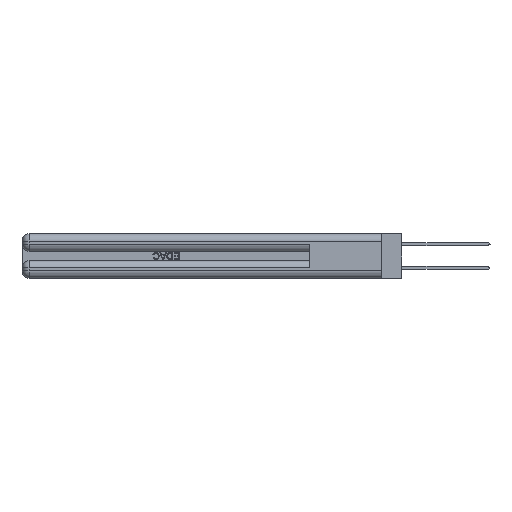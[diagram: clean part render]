
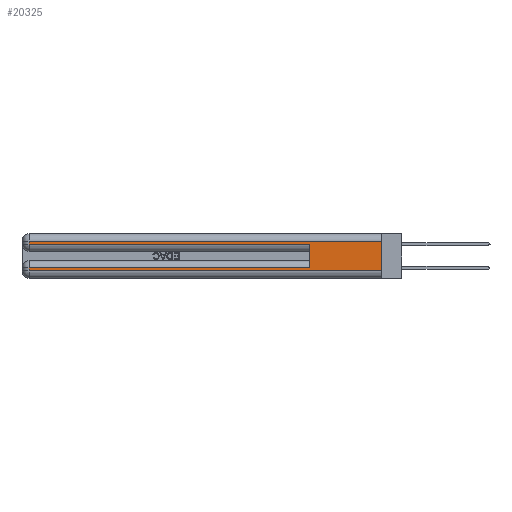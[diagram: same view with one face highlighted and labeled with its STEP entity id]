
A CAD part, left-side view. The second image highlights one B-rep face of the part: STEP entity #20325.
In plain terms, the highlighted planar face has unit normal (-1, 0, 0).
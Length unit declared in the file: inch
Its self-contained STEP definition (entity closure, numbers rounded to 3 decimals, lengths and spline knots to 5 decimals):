
#15 = CARTESIAN_POINT ( 'NONE',  ( 0., 0., 0.06 ) ) ;
#1481 = DIRECTION ( 'NONE',  ( 1., 0., 0. ) ) ;
#1722 = CARTESIAN_POINT ( 'NONE',  ( 0., 2.94, 0.085 ) ) ;
#2175 = LINE ( 'NONE', #39877, #17687 ) ;
#2631 = ORIENTED_EDGE ( 'NONE', *, *, #9699, .T. ) ;
#2966 = DIRECTION ( 'NONE',  ( 0., 1., 0. ) ) ;
#3398 = ORIENTED_EDGE ( 'NONE', *, *, #26807, .T. ) ;
#5607 = VECTOR ( 'NONE', #31214, 39.37008 ) ;
#5855 = ORIENTED_EDGE ( 'NONE', *, *, #34124, .F. ) ;
#5856 = VECTOR ( 'NONE', #18423, 39.37008 ) ;
#6084 = CARTESIAN_POINT ( 'NONE',  ( 0., 0., 0.31 ) ) ;
#6238 = DIRECTION ( 'NONE',  ( 0., 1., 0. ) ) ;
#6672 = ORIENTED_EDGE ( 'NONE', *, *, #23708, .F. ) ;
#8589 = DIRECTION ( 'NONE',  ( 0., -1., 0. ) ) ;
#9699 = EDGE_CURVE ( 'NONE', #20652, #22304, #37117, .T. ) ;
#9713 = EDGE_CURVE ( 'NONE', #44718, #11783, #11287, .T. ) ;
#11287 = LINE ( 'NONE', #19808, #5607 ) ;
#11373 = CARTESIAN_POINT ( 'NONE',  ( 0., 0.6, 0.145 ) ) ;
#11783 = VERTEX_POINT ( 'NONE', #21321 ) ;
#11836 = VECTOR ( 'NONE', #8589, 39.37008 ) ;
#13076 = EDGE_LOOP ( 'NONE', ( #5855, #37261, #20974, #2631, #6672, #3398, #45631, #32960 ) ) ;
#13133 = DIRECTION ( 'NONE',  ( 0., 0., -1. ) ) ;
#13942 = DIRECTION ( 'NONE',  ( 0., 0., 1. ) ) ;
#14789 = VECTOR ( 'NONE', #30973, 39.37008 ) ;
#15547 = VECTOR ( 'NONE', #6238, 39.37008 ) ;
#16800 = VERTEX_POINT ( 'NONE', #42448 ) ;
#17687 = VECTOR ( 'NONE', #13133, 39.37008 ) ;
#18271 = LINE ( 'NONE', #34170, #14789 ) ;
#18338 = VERTEX_POINT ( 'NONE', #30572 ) ;
#18423 = DIRECTION ( 'NONE',  ( 0., -1., 0. ) ) ;
#19808 = CARTESIAN_POINT ( 'NONE',  ( 0., 2.94, 0.37 ) ) ;
#19957 = PLANE ( 'NONE',  #35463 ) ;
#20325 = ADVANCED_FACE ( 'NONE', ( #29725 ), #19957, .F. ) ;
#20652 = VERTEX_POINT ( 'NONE', #40344 ) ;
#20974 = ORIENTED_EDGE ( 'NONE', *, *, #46164, .T. ) ;
#21218 = VERTEX_POINT ( 'NONE', #33392 ) ;
#21321 = CARTESIAN_POINT ( 'NONE',  ( 0., 2.94, 0.06 ) ) ;
#22148 = LINE ( 'NONE', #11373, #25037 ) ;
#22304 = VERTEX_POINT ( 'NONE', #31124 ) ;
#22329 = CARTESIAN_POINT ( 'NONE',  ( 0., 0., 0.31 ) ) ;
#23647 = DIRECTION ( 'NONE',  ( 0., 0., -1. ) ) ;
#23708 = EDGE_CURVE ( 'NONE', #21218, #22304, #22148, .T. ) ;
#25037 = VECTOR ( 'NONE', #13942, 39.37008 ) ;
#25139 = LINE ( 'NONE', #44872, #38830 ) ;
#26484 = LINE ( 'NONE', #15, #5856 ) ;
#26807 = EDGE_CURVE ( 'NONE', #21218, #44718, #25139, .T. ) ;
#29725 = FACE_OUTER_BOUND ( 'NONE', #13076, .T. ) ;
#30353 = EDGE_CURVE ( 'NONE', #11783, #16800, #26484, .T. ) ;
#30572 = CARTESIAN_POINT ( 'NONE',  ( 0., 2.94, 0.31 ) ) ;
#30973 = DIRECTION ( 'NONE',  ( 0., 0., -1. ) ) ;
#31124 = CARTESIAN_POINT ( 'NONE',  ( 0., 0.6, 0.285 ) ) ;
#31214 = DIRECTION ( 'NONE',  ( 0., 0., -1. ) ) ;
#32960 = ORIENTED_EDGE ( 'NONE', *, *, #30353, .T. ) ;
#33392 = CARTESIAN_POINT ( 'NONE',  ( 0., 0.6, 0.085 ) ) ;
#33419 = VERTEX_POINT ( 'NONE', #22329 ) ;
#34124 = EDGE_CURVE ( 'NONE', #33419, #16800, #18271, .T. ) ;
#34170 = CARTESIAN_POINT ( 'NONE',  ( 0., 0., 0.37 ) ) ;
#35091 = LINE ( 'NONE', #6084, #15547 ) ;
#35463 = AXIS2_PLACEMENT_3D ( 'NONE', #42029, #1481, #23647 ) ;
#37117 = LINE ( 'NONE', #38048, #11836 ) ;
#37261 = ORIENTED_EDGE ( 'NONE', *, *, #38712, .T. ) ;
#38048 = CARTESIAN_POINT ( 'NONE',  ( 0., 0., 0.285 ) ) ;
#38712 = EDGE_CURVE ( 'NONE', #33419, #18338, #35091, .T. ) ;
#38830 = VECTOR ( 'NONE', #2966, 39.37008 ) ;
#39877 = CARTESIAN_POINT ( 'NONE',  ( 0., 2.94, 0.37 ) ) ;
#40344 = CARTESIAN_POINT ( 'NONE',  ( 0., 2.94, 0.285 ) ) ;
#42029 = CARTESIAN_POINT ( 'NONE',  ( 0., 0., 0.37 ) ) ;
#42448 = CARTESIAN_POINT ( 'NONE',  ( 0., 0., 0.06 ) ) ;
#44718 = VERTEX_POINT ( 'NONE', #1722 ) ;
#44872 = CARTESIAN_POINT ( 'NONE',  ( 0., 0., 0.085 ) ) ;
#45631 = ORIENTED_EDGE ( 'NONE', *, *, #9713, .T. ) ;
#46164 = EDGE_CURVE ( 'NONE', #18338, #20652, #2175, .T. ) ;
